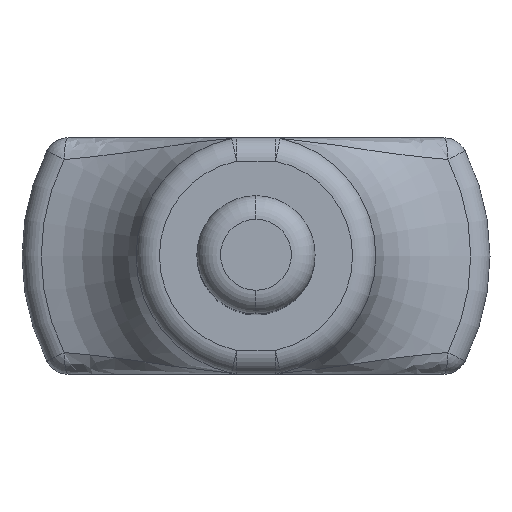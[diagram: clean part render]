
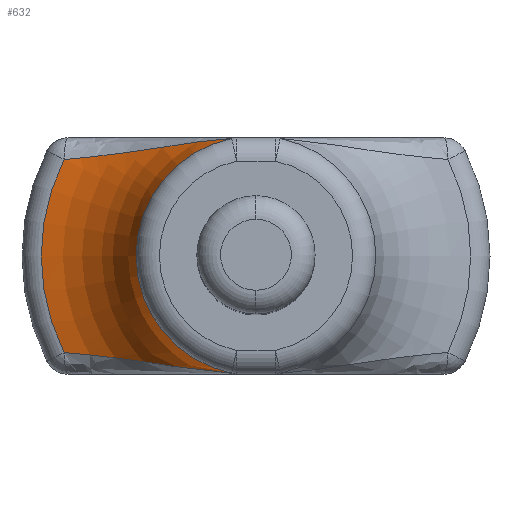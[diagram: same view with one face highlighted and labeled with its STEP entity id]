
A CAD part, top view. The second image highlights one B-rep face of the part: STEP entity #632.
In plain terms, the highlighted toroidal (fillet/blend) face has major radius 10 mm and minor radius 5 mm.
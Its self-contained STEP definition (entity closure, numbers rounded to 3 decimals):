
#69 = VERTEX_POINT ( 'NONE', #887 ) ;
#318 = AXIS2_PLACEMENT_3D ( 'NONE', #445, #444, #439 ) ;
#321 = AXIS2_PLACEMENT_3D ( 'NONE', #502, #531, #527 ) ;
#439 = DIRECTION ( 'NONE',  ( 0., -1., 0. ) ) ;
#444 = DIRECTION ( 'NONE',  ( 0., 0., 1. ) ) ;
#445 = CARTESIAN_POINT ( 'NONE',  ( 0., 2.522, -11.937 ) ) ;
#450 = CARTESIAN_POINT ( 'NONE',  ( -1.023, 7.487, -7.855 ) ) ;
#453 = CARTESIAN_POINT ( 'NONE',  ( -8.112, 6.604, -11.937 ) ) ;
#467 = CARTESIAN_POINT ( 'NONE',  ( -8.112, -1.561, -11.937 ) ) ;
#476 = CARTESIAN_POINT ( 'NONE',  ( -7.424, 6.664, -11.827 ) ) ;
#477 = CARTESIAN_POINT ( 'NONE',  ( -8.112, 6.604, -11.937 ) ) ;
#483 = CARTESIAN_POINT ( 'NONE',  ( -6.768, 6.732, -11.619 ) ) ;
#485 = CARTESIAN_POINT ( 'NONE',  ( -5.819, 6.849, -11.205 ) ) ;
#492 = CARTESIAN_POINT ( 'NONE',  ( -5.508, 6.89, -11.05 ) ) ;
#502 = CARTESIAN_POINT ( 'NONE',  ( 0., 2.522, -7.855 ) ) ;
#506 = CARTESIAN_POINT ( 'NONE',  ( -3.748, 7.15, -9.977 ) ) ;
#507 = CARTESIAN_POINT ( 'NONE',  ( -4.905, 6.975, -10.717 ) ) ;
#516 = CARTESIAN_POINT ( 'NONE',  ( -4.612, 7.018, -10.538 ) ) ;
#522 = CARTESIAN_POINT ( 'NONE',  ( -3.194, 7.238, -9.569 ) ) ;
#524 = CARTESIAN_POINT ( 'NONE',  ( -1.023, 7.487, -7.855 ) ) ;
#527 = DIRECTION ( 'NONE',  ( 0., -1., 0. ) ) ;
#531 = DIRECTION ( 'NONE',  ( 0., 0., -1. ) ) ;
#541 = CARTESIAN_POINT ( 'NONE',  ( -2.1, 7.39, -8.726 ) ) ;
#543 = CARTESIAN_POINT ( 'NONE',  ( -1.561, 7.452, -8.292 ) ) ;
#544 = CARTESIAN_POINT ( 'NONE',  ( -3.748, -2.106, -9.977 ) ) ;
#563 = CARTESIAN_POINT ( 'NONE',  ( -1.023, -2.444, -7.855 ) ) ;
#576 = CARTESIAN_POINT ( 'NONE',  ( -2.1, -2.346, -8.726 ) ) ;
#577 = CARTESIAN_POINT ( 'NONE',  ( -1.561, -2.409, -8.292 ) ) ;
#581 = AXIS2_PLACEMENT_3D ( 'NONE', #853, #876, #863 ) ;
#595 = CARTESIAN_POINT ( 'NONE',  ( -3.194, -2.195, -9.569 ) ) ;
#608 = CARTESIAN_POINT ( 'NONE',  ( -4.612, -1.975, -10.538 ) ) ;
#612 = CARTESIAN_POINT ( 'NONE',  ( -5.508, -1.847, -11.05 ) ) ;
#619 = CARTESIAN_POINT ( 'NONE',  ( -6.768, -1.689, -11.619 ) ) ;
#621 = CARTESIAN_POINT ( 'NONE',  ( -4.905, -1.931, -10.717 ) ) ;
#624 = CARTESIAN_POINT ( 'NONE',  ( -5.819, -1.805, -11.205 ) ) ;
#625 = CARTESIAN_POINT ( 'NONE',  ( -7.424, -1.62, -11.827 ) ) ;
#632 = ADVANCED_FACE ( 'NONE', ( #823 ), #821, .F. ) ;
#642 = CARTESIAN_POINT ( 'NONE',  ( -8.112, -1.561, -11.937 ) ) ;
#713 = CIRCLE ( 'NONE', #321, 5.07 ) ;
#723 = CIRCLE ( 'NONE', #318, 9.082 ) ;
#821 = TOROIDAL_SURFACE ( 'NONE', #581, 10., 5. ) ;
#823 = FACE_OUTER_BOUND ( 'NONE', #1255, .T. ) ;
#853 = CARTESIAN_POINT ( 'NONE',  ( 0., 2.522, -7.022 ) ) ;
#863 = DIRECTION ( 'NONE',  ( 0., 1., 0. ) ) ;
#876 = DIRECTION ( 'NONE',  ( 0., 0., -1. ) ) ;
#887 = CARTESIAN_POINT ( 'NONE',  ( -1.023, -2.444, -7.855 ) ) ;
#955 = ORIENTED_EDGE ( 'NONE', *, *, #985, .T. ) ;
#957 = ORIENTED_EDGE ( 'NONE', *, *, #987, .T. ) ;
#960 = ORIENTED_EDGE ( 'NONE', *, *, #994, .T. ) ;
#985 = EDGE_CURVE ( 'NONE', #1232, #69, #1228, .T. ) ;
#987 = EDGE_CURVE ( 'NONE', #69, #1280, #713, .T. ) ;
#994 = EDGE_CURVE ( 'NONE', #1280, #1271, #1227, .T. ) ;
#995 = EDGE_CURVE ( 'NONE', #1271, #1232, #723, .T. ) ;
#1012 = ORIENTED_EDGE ( 'NONE', *, *, #995, .T. ) ;
#1227 = B_SPLINE_CURVE_WITH_KNOTS ( 'NONE', 3,
 ( #524, #543, #541, #522, #506, #516, #507, #492, #485, #483, #476, #477 ),
 .UNSPECIFIED., .F., .F.,
 ( 4, 2, 2, 2, 2, 4 ),
 ( 0.001, 0.003, 0.005, 0.007, 0.008, 0.01 ),
 .UNSPECIFIED. ) ;
#1228 = B_SPLINE_CURVE_WITH_KNOTS ( 'NONE', 3,
 ( #642, #625, #619, #624, #612, #621, #608, #544, #595, #576, #577, #563 ),
 .UNSPECIFIED., .F., .F.,
 ( 4, 2, 2, 2, 2, 4 ),
 ( 0., 0.002, 0.003, 0.004, 0.006, 0.008 ),
 .UNSPECIFIED. ) ;
#1232 = VERTEX_POINT ( 'NONE', #467 ) ;
#1255 = EDGE_LOOP ( 'NONE', ( #955, #957, #960, #1012 ) ) ;
#1271 = VERTEX_POINT ( 'NONE', #453 ) ;
#1280 = VERTEX_POINT ( 'NONE', #450 ) ;
